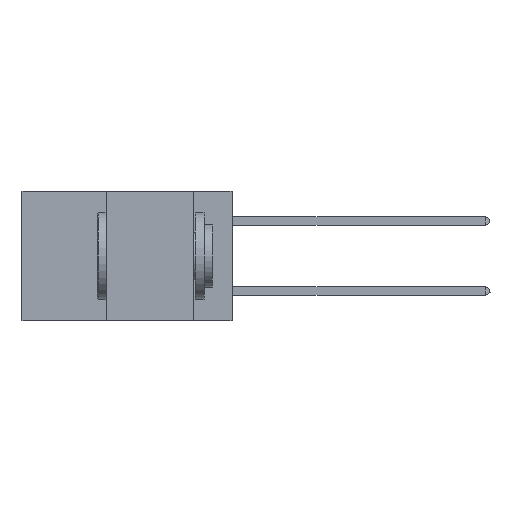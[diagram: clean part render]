
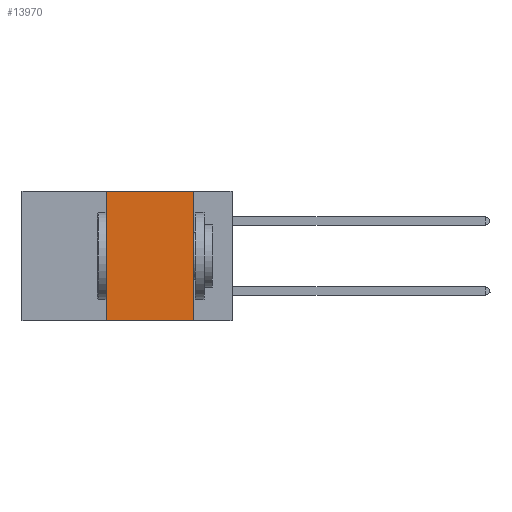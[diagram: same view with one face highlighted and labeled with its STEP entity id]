
A CAD part, left-side view. The second image highlights one B-rep face of the part: STEP entity #13970.
In plain terms, the highlighted planar face has unit normal (-1, 0, 0).
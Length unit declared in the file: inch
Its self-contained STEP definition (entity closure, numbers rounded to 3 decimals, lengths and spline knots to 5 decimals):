
#267 = CARTESIAN_POINT ( 'NONE',  ( 0., 0.6, -0.37 ) ) ;
#360 = DIRECTION ( 'NONE',  ( 0., 0., -1. ) ) ;
#729 = FACE_OUTER_BOUND ( 'NONE', #21686, .T. ) ;
#805 = VECTOR ( 'NONE', #360, 39.37008 ) ;
#2917 = VERTEX_POINT ( 'NONE', #4987 ) ;
#3079 = DIRECTION ( 'NONE',  ( 0., -1., 0. ) ) ;
#4268 = LINE ( 'NONE', #10218, #17032 ) ;
#4987 = CARTESIAN_POINT ( 'NONE',  ( 0., 0.36, -0.37 ) ) ;
#6215 = EDGE_CURVE ( 'NONE', #2917, #17726, #26533, .T. ) ;
#6563 = CARTESIAN_POINT ( 'NONE',  ( 0., 0.6, 0. ) ) ;
#6812 = LINE ( 'NONE', #31354, #805 ) ;
#7316 = VECTOR ( 'NONE', #3079, 39.37008 ) ;
#8214 = CARTESIAN_POINT ( 'NONE',  ( 0., 0.36, 0. ) ) ;
#9279 = DIRECTION ( 'NONE',  ( 0., 0., -1. ) ) ;
#10218 = CARTESIAN_POINT ( 'NONE',  ( 0., 0.6, 0. ) ) ;
#12378 = ORIENTED_EDGE ( 'NONE', *, *, #17270, .T. ) ;
#13127 = DIRECTION ( 'NONE',  ( 0., 0., 1. ) ) ;
#13970 = ADVANCED_FACE ( 'NONE', ( #729 ), #31961, .F. ) ;
#15512 = CARTESIAN_POINT ( 'NONE',  ( 0., 0.11, 0. ) ) ;
#17032 = VECTOR ( 'NONE', #22919, 39.37008 ) ;
#17270 = EDGE_CURVE ( 'NONE', #2917, #17573, #17328, .T. ) ;
#17328 = LINE ( 'NONE', #267, #7316 ) ;
#17573 = VERTEX_POINT ( 'NONE', #24678 ) ;
#17726 = VERTEX_POINT ( 'NONE', #22305 ) ;
#18439 = EDGE_CURVE ( 'NONE', #32262, #17573, #6812, .T. ) ;
#21686 = EDGE_LOOP ( 'NONE', ( #30933, #27455, #23316, #12378 ) ) ;
#22305 = CARTESIAN_POINT ( 'NONE',  ( 0., 0.36, 0. ) ) ;
#22919 = DIRECTION ( 'NONE',  ( 0., -1., 0. ) ) ;
#23316 = ORIENTED_EDGE ( 'NONE', *, *, #6215, .F. ) ;
#24094 = VECTOR ( 'NONE', #13127, 39.37008 ) ;
#24244 = DIRECTION ( 'NONE',  ( 1., 0., 0. ) ) ;
#24343 = AXIS2_PLACEMENT_3D ( 'NONE', #6563, #24244, #9279 ) ;
#24678 = CARTESIAN_POINT ( 'NONE',  ( 0., 0.11, -0.37 ) ) ;
#26533 = LINE ( 'NONE', #8214, #24094 ) ;
#27455 = ORIENTED_EDGE ( 'NONE', *, *, #30497, .F. ) ;
#30497 = EDGE_CURVE ( 'NONE', #17726, #32262, #4268, .T. ) ;
#30933 = ORIENTED_EDGE ( 'NONE', *, *, #18439, .F. ) ;
#31354 = CARTESIAN_POINT ( 'NONE',  ( 0., 0.11, 0. ) ) ;
#31961 = PLANE ( 'NONE',  #24343 ) ;
#32262 = VERTEX_POINT ( 'NONE', #15512 ) ;
